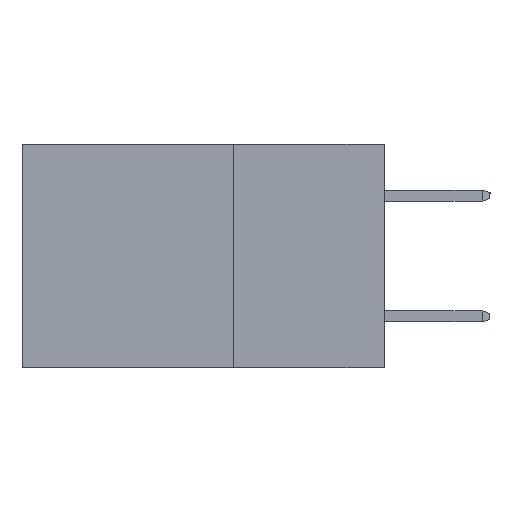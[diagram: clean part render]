
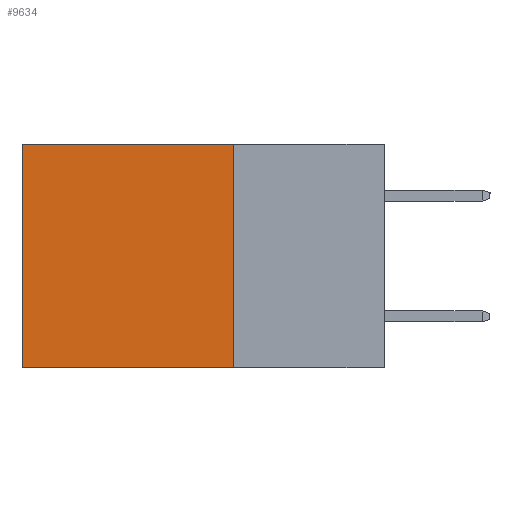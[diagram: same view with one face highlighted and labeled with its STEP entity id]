
A CAD part, left-side view. The second image highlights one B-rep face of the part: STEP entity #9634.
In plain terms, the highlighted planar face has unit normal (-1, 0, 0).
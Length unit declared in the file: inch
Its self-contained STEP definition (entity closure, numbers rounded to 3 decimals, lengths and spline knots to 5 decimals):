
#1551 = CARTESIAN_POINT ( 'NONE',  ( 0.2615, 0.25, 0. ) ) ;
#2366 = VECTOR ( 'NONE', #9045, 39.37008 ) ;
#3306 = DIRECTION ( 'NONE',  ( 0., 0., -1. ) ) ;
#3720 = VERTEX_POINT ( 'NONE', #1551 ) ;
#3740 = FACE_OUTER_BOUND ( 'NONE', #10504, .T. ) ;
#4160 = CARTESIAN_POINT ( 'NONE',  ( 0.2615, 0.6, -0.37 ) ) ;
#5193 = EDGE_CURVE ( 'NONE', #12197, #8578, #16546, .T. ) ;
#5410 = EDGE_CURVE ( 'NONE', #3720, #12173, #18456, .T. ) ;
#5506 = CARTESIAN_POINT ( 'NONE',  ( 0.2615, 0.25, -0.37 ) ) ;
#6616 = ORIENTED_EDGE ( 'NONE', *, *, #24084, .F. ) ;
#6868 = LINE ( 'NONE', #10556, #6947 ) ;
#6947 = VECTOR ( 'NONE', #3306, 39.37008 ) ;
#7236 = DIRECTION ( 'NONE',  ( 0., 1., 0. ) ) ;
#7517 = VECTOR ( 'NONE', #12387, 39.37008 ) ;
#7560 = CARTESIAN_POINT ( 'NONE',  ( 0.2615, 0.25, -0.37 ) ) ;
#8578 = VERTEX_POINT ( 'NONE', #4160 ) ;
#9045 = DIRECTION ( 'NONE',  ( 0., 1., 0. ) ) ;
#9634 = ADVANCED_FACE ( 'NONE', ( #3740 ), #11221, .F. ) ;
#9749 = DIRECTION ( 'NONE',  ( 1., 0., 0. ) ) ;
#10425 = LINE ( 'NONE', #17872, #7517 ) ;
#10475 = ORIENTED_EDGE ( 'NONE', *, *, #5193, .F. ) ;
#10504 = EDGE_LOOP ( 'NONE', ( #11661, #10475, #6616, #17621 ) ) ;
#10556 = CARTESIAN_POINT ( 'NONE',  ( 0.2615, 0.25, -0.37 ) ) ;
#11221 = PLANE ( 'NONE',  #15146 ) ;
#11661 = ORIENTED_EDGE ( 'NONE', *, *, #18941, .T. ) ;
#12173 = VERTEX_POINT ( 'NONE', #16330 ) ;
#12197 = VERTEX_POINT ( 'NONE', #19996 ) ;
#12387 = DIRECTION ( 'NONE',  ( 0., 0., -1. ) ) ;
#15146 = AXIS2_PLACEMENT_3D ( 'NONE', #7560, #9749, #17565 ) ;
#16330 = CARTESIAN_POINT ( 'NONE',  ( 0.2615, 0.6, 0. ) ) ;
#16546 = LINE ( 'NONE', #5506, #19564 ) ;
#17565 = DIRECTION ( 'NONE',  ( 0., 0., -1. ) ) ;
#17621 = ORIENTED_EDGE ( 'NONE', *, *, #5410, .T. ) ;
#17872 = CARTESIAN_POINT ( 'NONE',  ( 0.2615, 0.6, -0.37 ) ) ;
#18456 = LINE ( 'NONE', #21653, #2366 ) ;
#18941 = EDGE_CURVE ( 'NONE', #12173, #8578, #10425, .T. ) ;
#19564 = VECTOR ( 'NONE', #7236, 39.37008 ) ;
#19996 = CARTESIAN_POINT ( 'NONE',  ( 0.2615, 0.25, -0.37 ) ) ;
#21653 = CARTESIAN_POINT ( 'NONE',  ( 0.2615, 0.25, 0. ) ) ;
#24084 = EDGE_CURVE ( 'NONE', #3720, #12197, #6868, .T. ) ;
